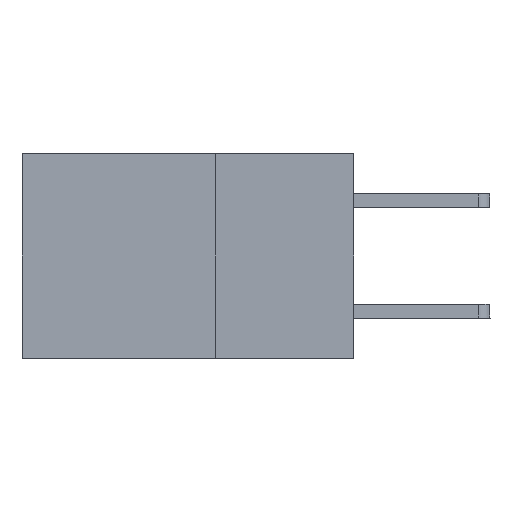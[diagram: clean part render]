
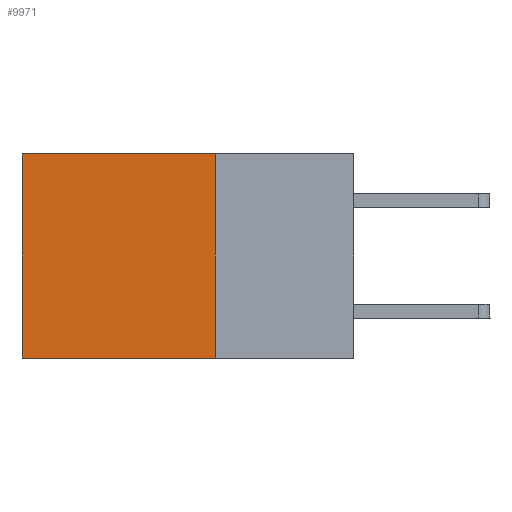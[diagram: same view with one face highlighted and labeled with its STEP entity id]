
A CAD part, left-side view. The second image highlights one B-rep face of the part: STEP entity #9971.
In plain terms, the highlighted planar face has unit normal (-1, 0, 0).
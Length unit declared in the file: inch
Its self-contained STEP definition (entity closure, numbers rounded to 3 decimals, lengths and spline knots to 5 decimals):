
#30 = LINE ( 'NONE', #10587, #2341 ) ;
#262 = CARTESIAN_POINT ( 'NONE',  ( 0.2875, 0.25, 0. ) ) ;
#372 = ORIENTED_EDGE ( 'NONE', *, *, #8877, .T. ) ;
#1059 = ORIENTED_EDGE ( 'NONE', *, *, #2068, .F. ) ;
#1493 = EDGE_LOOP ( 'NONE', ( #372, #1059, #10885, #4871 ) ) ;
#1804 = CARTESIAN_POINT ( 'NONE',  ( 0.2875, 0.6, -0.37 ) ) ;
#2068 = EDGE_CURVE ( 'NONE', #8011, #9640, #11061, .T. ) ;
#2341 = VECTOR ( 'NONE', #10422, 39.37008 ) ;
#2697 = EDGE_CURVE ( 'NONE', #2748, #8011, #10596, .T. ) ;
#2748 = VERTEX_POINT ( 'NONE', #9684 ) ;
#3072 = VECTOR ( 'NONE', #9840, 39.37008 ) ;
#3273 = DIRECTION ( 'NONE',  ( 0., 1., 0. ) ) ;
#4647 = VERTEX_POINT ( 'NONE', #9297 ) ;
#4871 = ORIENTED_EDGE ( 'NONE', *, *, #8739, .T. ) ;
#4951 = PLANE ( 'NONE',  #9633 ) ;
#6314 = VECTOR ( 'NONE', #8078, 39.37008 ) ;
#6434 = CARTESIAN_POINT ( 'NONE',  ( 0.2875, 0.25, -0.37 ) ) ;
#6823 = CARTESIAN_POINT ( 'NONE',  ( 0.2875, 0.25, 0. ) ) ;
#7032 = VECTOR ( 'NONE', #3273, 39.37008 ) ;
#7357 = CARTESIAN_POINT ( 'NONE',  ( 0.2875, 0.25, -0.37 ) ) ;
#7569 = DIRECTION ( 'NONE',  ( 0., 0., -1. ) ) ;
#8011 = VERTEX_POINT ( 'NONE', #6434 ) ;
#8078 = DIRECTION ( 'NONE',  ( 0., 0., -1. ) ) ;
#8739 = EDGE_CURVE ( 'NONE', #2748, #4647, #30, .T. ) ;
#8877 = EDGE_CURVE ( 'NONE', #4647, #9640, #10639, .T. ) ;
#9297 = CARTESIAN_POINT ( 'NONE',  ( 0.2875, 0.6, 0. ) ) ;
#9633 = AXIS2_PLACEMENT_3D ( 'NONE', #6823, #10983, #7569 ) ;
#9640 = VERTEX_POINT ( 'NONE', #1804 ) ;
#9684 = CARTESIAN_POINT ( 'NONE',  ( 0.2875, 0.25, 0. ) ) ;
#9840 = DIRECTION ( 'NONE',  ( 0., 0., -1. ) ) ;
#9891 = CARTESIAN_POINT ( 'NONE',  ( 0.2875, 0.6, 0. ) ) ;
#9971 = ADVANCED_FACE ( 'NONE', ( #10367 ), #4951, .F. ) ;
#10367 = FACE_OUTER_BOUND ( 'NONE', #1493, .T. ) ;
#10422 = DIRECTION ( 'NONE',  ( 0., 1., 0. ) ) ;
#10587 = CARTESIAN_POINT ( 'NONE',  ( 0.2875, 0.25, 0. ) ) ;
#10596 = LINE ( 'NONE', #262, #6314 ) ;
#10639 = LINE ( 'NONE', #9891, #3072 ) ;
#10885 = ORIENTED_EDGE ( 'NONE', *, *, #2697, .F. ) ;
#10983 = DIRECTION ( 'NONE',  ( 1., 0., 0. ) ) ;
#11061 = LINE ( 'NONE', #7357, #7032 ) ;
